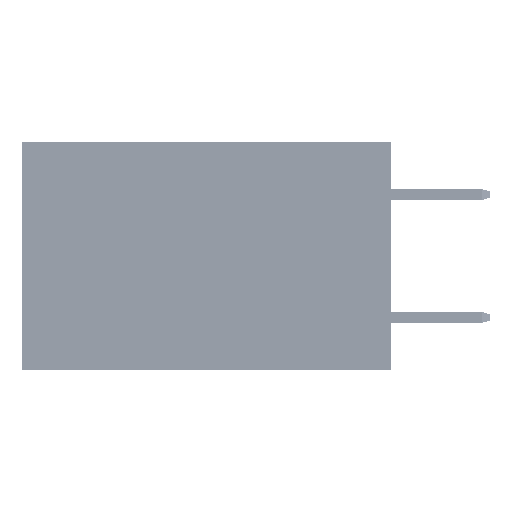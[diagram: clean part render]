
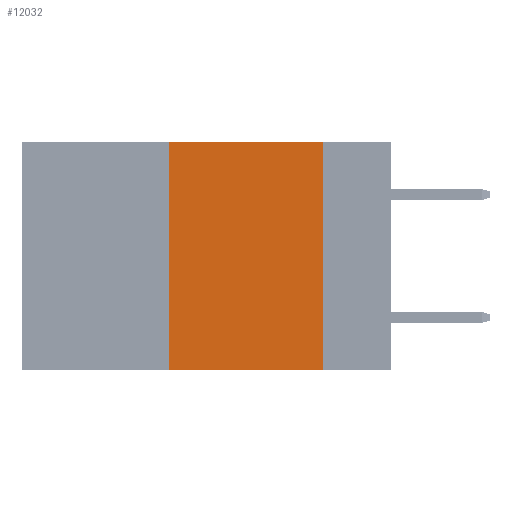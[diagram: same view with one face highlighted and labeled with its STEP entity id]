
A CAD part, left-side view. The second image highlights one B-rep face of the part: STEP entity #12032.
In plain terms, the highlighted planar face has unit normal (-1, 0, 0).
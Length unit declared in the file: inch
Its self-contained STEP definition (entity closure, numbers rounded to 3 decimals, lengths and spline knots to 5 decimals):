
#252 = VECTOR ( 'NONE', #20287, 39.37008 ) ;
#285 = VERTEX_POINT ( 'NONE', #40568 ) ;
#1361 = DIRECTION ( 'NONE',  ( 0., 0., 1. ) ) ;
#2624 = CARTESIAN_POINT ( 'NONE',  ( 0., 0.11, 0. ) ) ;
#4846 = AXIS2_PLACEMENT_3D ( 'NONE', #42956, #20189, #24037 ) ;
#10639 = FACE_OUTER_BOUND ( 'NONE', #39112, .T. ) ;
#12032 = ADVANCED_FACE ( 'NONE', ( #10639 ), #24193, .F. ) ;
#14881 = EDGE_CURVE ( 'NONE', #30517, #34602, #47419, .T. ) ;
#16101 = ORIENTED_EDGE ( 'NONE', *, *, #33575, .T. ) ;
#20024 = EDGE_CURVE ( 'NONE', #285, #30517, #45609, .T. ) ;
#20189 = DIRECTION ( 'NONE',  ( 1., 0., 0. ) ) ;
#20287 = DIRECTION ( 'NONE',  ( 0., -1., 0. ) ) ;
#20620 = CARTESIAN_POINT ( 'NONE',  ( 0., 0.6, -0.37 ) ) ;
#23392 = ORIENTED_EDGE ( 'NONE', *, *, #20024, .F. ) ;
#24037 = DIRECTION ( 'NONE',  ( 0., 0., -1. ) ) ;
#24193 = PLANE ( 'NONE',  #4846 ) ;
#25573 = CARTESIAN_POINT ( 'NONE',  ( 0., 0.11, -0.37 ) ) ;
#27195 = ORIENTED_EDGE ( 'NONE', *, *, #14881, .F. ) ;
#28446 = CARTESIAN_POINT ( 'NONE',  ( 0., 0.36, 0. ) ) ;
#28817 = ORIENTED_EDGE ( 'NONE', *, *, #47745, .F. ) ;
#30517 = VERTEX_POINT ( 'NONE', #36427 ) ;
#32512 = VERTEX_POINT ( 'NONE', #32988 ) ;
#32988 = CARTESIAN_POINT ( 'NONE',  ( 0., 0.36, -0.37 ) ) ;
#33575 = EDGE_CURVE ( 'NONE', #32512, #34602, #40897, .T. ) ;
#34165 = DIRECTION ( 'NONE',  ( 0., 0., -1. ) ) ;
#34602 = VERTEX_POINT ( 'NONE', #25573 ) ;
#35471 = VECTOR ( 'NONE', #40991, 39.37008 ) ;
#36427 = CARTESIAN_POINT ( 'NONE',  ( 0., 0.11, 0. ) ) ;
#37230 = VECTOR ( 'NONE', #1361, 39.37008 ) ;
#39112 = EDGE_LOOP ( 'NONE', ( #27195, #23392, #28817, #16101 ) ) ;
#40216 = LINE ( 'NONE', #28446, #37230 ) ;
#40333 = CARTESIAN_POINT ( 'NONE',  ( 0., 0.6, 0. ) ) ;
#40568 = CARTESIAN_POINT ( 'NONE',  ( 0., 0.36, 0. ) ) ;
#40897 = LINE ( 'NONE', #20620, #252 ) ;
#40991 = DIRECTION ( 'NONE',  ( 0., -1., 0. ) ) ;
#42956 = CARTESIAN_POINT ( 'NONE',  ( 0., 0.6, 0. ) ) ;
#45019 = VECTOR ( 'NONE', #34165, 39.37008 ) ;
#45609 = LINE ( 'NONE', #40333, #35471 ) ;
#47419 = LINE ( 'NONE', #2624, #45019 ) ;
#47745 = EDGE_CURVE ( 'NONE', #32512, #285, #40216, .T. ) ;
